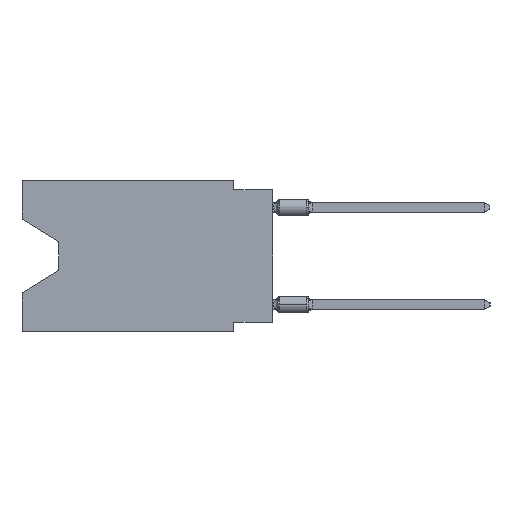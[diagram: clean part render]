
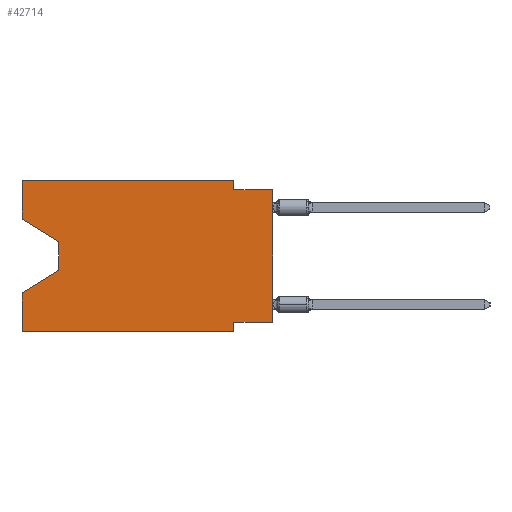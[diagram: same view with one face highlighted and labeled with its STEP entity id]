
A CAD part, left-side view. The second image highlights one B-rep face of the part: STEP entity #42714.
In plain terms, the highlighted planar face has unit normal (-1, 0, 0).
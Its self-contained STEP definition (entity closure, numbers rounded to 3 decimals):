
#703 = DIRECTION ( 'NONE',  ( 0., 0., 1. ) ) ;
#1311 = CARTESIAN_POINT ( 'NONE',  ( 0., 2.54, 0. ) ) ;
#2325 = ORIENTED_EDGE ( 'NONE', *, *, #37744, .F. ) ;
#3417 = CARTESIAN_POINT ( 'NONE',  ( 0., 13.97, -5.893 ) ) ;
#3583 = LINE ( 'NONE', #37538, #43249 ) ;
#3723 = LINE ( 'NONE', #6797, #4018 ) ;
#4018 = VECTOR ( 'NONE', #41042, 1000. ) ;
#5002 = LINE ( 'NONE', #22260, #16687 ) ;
#5147 = LINE ( 'NONE', #21572, #17436 ) ;
#5510 = EDGE_LOOP ( 'NONE', ( #19944, #20531, #32847, #5876, #44798, #30963, #9628, #25011, #17521, #24845, #2325, #19287 ) ) ;
#5648 = DIRECTION ( 'NONE',  ( 0., -0.855, -0.519 ) ) ;
#5876 = ORIENTED_EDGE ( 'NONE', *, *, #41358, .F. ) ;
#6670 = VECTOR ( 'NONE', #16341, 1000. ) ;
#6797 = CARTESIAN_POINT ( 'NONE',  ( 0., 16.383, -9.906 ) ) ;
#6939 = DIRECTION ( 'NONE',  ( 0., 0., -1. ) ) ;
#7843 = EDGE_CURVE ( 'NONE', #8229, #17250, #5002, .T. ) ;
#8229 = VERTEX_POINT ( 'NONE', #30304 ) ;
#8621 = VERTEX_POINT ( 'NONE', #48214 ) ;
#9628 = ORIENTED_EDGE ( 'NONE', *, *, #16466, .F. ) ;
#9954 = VERTEX_POINT ( 'NONE', #10150 ) ;
#10150 = CARTESIAN_POINT ( 'NONE',  ( 0., 13.97, -5.893 ) ) ;
#10345 = EDGE_CURVE ( 'NONE', #41089, #18686, #43511, .T. ) ;
#10694 = CARTESIAN_POINT ( 'NONE',  ( 0., 0., -0.635 ) ) ;
#10838 = FACE_OUTER_BOUND ( 'NONE', #5510, .T. ) ;
#11497 = CARTESIAN_POINT ( 'NONE',  ( 0., 13.97, -4.013 ) ) ;
#11976 = CARTESIAN_POINT ( 'NONE',  ( 0., 2.54, -9.906 ) ) ;
#12316 = DIRECTION ( 'NONE',  ( 0., 0., 1. ) ) ;
#13306 = VERTEX_POINT ( 'NONE', #29575 ) ;
#13396 = EDGE_CURVE ( 'NONE', #9954, #23863, #41544, .T. ) ;
#13417 = VECTOR ( 'NONE', #31026, 1000. ) ;
#14428 = EDGE_CURVE ( 'NONE', #17956, #8621, #48243, .T. ) ;
#15875 = VECTOR ( 'NONE', #5648, 1000. ) ;
#16341 = DIRECTION ( 'NONE',  ( 0., -1., 0. ) ) ;
#16466 = EDGE_CURVE ( 'NONE', #23738, #8229, #34900, .T. ) ;
#16520 = CARTESIAN_POINT ( 'NONE',  ( 0., 16.383, 0. ) ) ;
#16586 = EDGE_CURVE ( 'NONE', #8621, #9954, #41009, .T. ) ;
#16687 = VECTOR ( 'NONE', #35064, 1000. ) ;
#17250 = VERTEX_POINT ( 'NONE', #11976 ) ;
#17436 = VECTOR ( 'NONE', #703, 1000. ) ;
#17521 = ORIENTED_EDGE ( 'NONE', *, *, #23000, .F. ) ;
#17905 = CARTESIAN_POINT ( 'NONE',  ( 0., 16.383, -2.546 ) ) ;
#17956 = VERTEX_POINT ( 'NONE', #28017 ) ;
#18455 = CARTESIAN_POINT ( 'NONE',  ( 0., 0., -9.271 ) ) ;
#18686 = VERTEX_POINT ( 'NONE', #35532 ) ;
#19287 = ORIENTED_EDGE ( 'NONE', *, *, #26984, .F. ) ;
#19826 = DIRECTION ( 'NONE',  ( 0., 0.855, -0.519 ) ) ;
#19944 = ORIENTED_EDGE ( 'NONE', *, *, #14428, .T. ) ;
#20531 = ORIENTED_EDGE ( 'NONE', *, *, #16586, .T. ) ;
#21572 = CARTESIAN_POINT ( 'NONE',  ( 0., 16.383, 0. ) ) ;
#22260 = CARTESIAN_POINT ( 'NONE',  ( 0., 2.54, -9.906 ) ) ;
#22882 = AXIS2_PLACEMENT_3D ( 'NONE', #53996, #23648, #6939 ) ;
#23000 = EDGE_CURVE ( 'NONE', #18686, #36384, #33600, .T. ) ;
#23189 = VERTEX_POINT ( 'NONE', #42765 ) ;
#23648 = DIRECTION ( 'NONE',  ( 1., 0., 0. ) ) ;
#23738 = VERTEX_POINT ( 'NONE', #18455 ) ;
#23863 = VERTEX_POINT ( 'NONE', #28493 ) ;
#24845 = ORIENTED_EDGE ( 'NONE', *, *, #10345, .F. ) ;
#25011 = ORIENTED_EDGE ( 'NONE', *, *, #29064, .T. ) ;
#25154 = LINE ( 'NONE', #16520, #27716 ) ;
#26984 = EDGE_CURVE ( 'NONE', #17956, #23189, #33215, .T. ) ;
#27716 = VECTOR ( 'NONE', #28540, 1000. ) ;
#27839 = PLANE ( 'NONE',  #22882 ) ;
#28017 = CARTESIAN_POINT ( 'NONE',  ( 0., 16.383, -2.546 ) ) ;
#28493 = CARTESIAN_POINT ( 'NONE',  ( 0., 16.383, -7.36 ) ) ;
#28540 = DIRECTION ( 'NONE',  ( 0., -1., 0. ) ) ;
#29064 = EDGE_CURVE ( 'NONE', #23738, #36384, #3583, .T. ) ;
#29575 = CARTESIAN_POINT ( 'NONE',  ( 0., 16.383, -9.906 ) ) ;
#30304 = CARTESIAN_POINT ( 'NONE',  ( 0., 2.54, -9.271 ) ) ;
#30963 = ORIENTED_EDGE ( 'NONE', *, *, #7843, .F. ) ;
#31026 = DIRECTION ( 'NONE',  ( 0., 1., 0. ) ) ;
#32309 = DIRECTION ( 'NONE',  ( 0., 0., -1. ) ) ;
#32847 = ORIENTED_EDGE ( 'NONE', *, *, #13396, .T. ) ;
#33048 = VECTOR ( 'NONE', #44904, 1000. ) ;
#33215 = LINE ( 'NONE', #54910, #36778 ) ;
#33460 = VECTOR ( 'NONE', #32309, 1000. ) ;
#33600 = LINE ( 'NONE', #45323, #6670 ) ;
#34881 = CARTESIAN_POINT ( 'NONE',  ( 0., 2.54, 0. ) ) ;
#34900 = LINE ( 'NONE', #48250, #13417 ) ;
#35064 = DIRECTION ( 'NONE',  ( 0., 0., -1. ) ) ;
#35532 = CARTESIAN_POINT ( 'NONE',  ( 0., 2.54, -0.635 ) ) ;
#36384 = VERTEX_POINT ( 'NONE', #10694 ) ;
#36778 = VECTOR ( 'NONE', #12316, 1000. ) ;
#37538 = CARTESIAN_POINT ( 'NONE',  ( 0., 0., 0. ) ) ;
#37744 = EDGE_CURVE ( 'NONE', #23189, #41089, #25154, .T. ) ;
#41009 = LINE ( 'NONE', #11497, #33048 ) ;
#41042 = DIRECTION ( 'NONE',  ( 0., -1., 0. ) ) ;
#41089 = VERTEX_POINT ( 'NONE', #1311 ) ;
#41358 = EDGE_CURVE ( 'NONE', #13306, #23863, #5147, .T. ) ;
#41544 = LINE ( 'NONE', #3417, #47787 ) ;
#42714 = ADVANCED_FACE ( 'NONE', ( #10838 ), #27839, .F. ) ;
#42765 = CARTESIAN_POINT ( 'NONE',  ( 0., 16.383, 0. ) ) ;
#43249 = VECTOR ( 'NONE', #45616, 1000. ) ;
#43511 = LINE ( 'NONE', #34881, #33460 ) ;
#44798 = ORIENTED_EDGE ( 'NONE', *, *, #51875, .T. ) ;
#44904 = DIRECTION ( 'NONE',  ( 0., 0., -1. ) ) ;
#45323 = CARTESIAN_POINT ( 'NONE',  ( 0., 0., -0.635 ) ) ;
#45616 = DIRECTION ( 'NONE',  ( 0., 0., 1. ) ) ;
#47787 = VECTOR ( 'NONE', #19826, 1000. ) ;
#48214 = CARTESIAN_POINT ( 'NONE',  ( 0., 13.97, -4.013 ) ) ;
#48243 = LINE ( 'NONE', #17905, #15875 ) ;
#48250 = CARTESIAN_POINT ( 'NONE',  ( 0., 0., -9.271 ) ) ;
#51875 = EDGE_CURVE ( 'NONE', #13306, #17250, #3723, .T. ) ;
#53996 = CARTESIAN_POINT ( 'NONE',  ( 0., 16.383, 0. ) ) ;
#54910 = CARTESIAN_POINT ( 'NONE',  ( 0., 16.383, 0. ) ) ;
